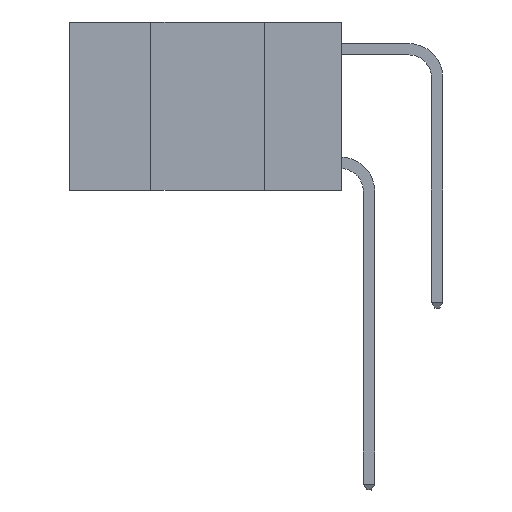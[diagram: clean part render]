
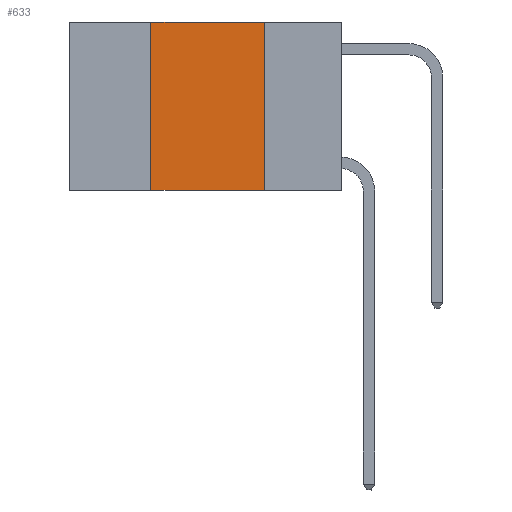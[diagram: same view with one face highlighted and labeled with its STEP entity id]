
A CAD part, left-side view. The second image highlights one B-rep face of the part: STEP entity #633.
In plain terms, the highlighted planar face has unit normal (-1, 0, 0).
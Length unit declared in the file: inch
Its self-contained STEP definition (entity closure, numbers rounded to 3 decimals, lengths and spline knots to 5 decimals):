
#192 = VECTOR ( 'NONE', #5449, 39.37008 ) ;
#633 = ADVANCED_FACE ( 'NONE', ( #22563 ), #10099, .F. ) ;
#636 = CARTESIAN_POINT ( 'NONE',  ( 0., 0.6, -0.37 ) ) ;
#1644 = DIRECTION ( 'NONE',  ( 0., 0., 1. ) ) ;
#1750 = LINE ( 'NONE', #636, #192 ) ;
#2427 = EDGE_CURVE ( 'NONE', #15193, #10401, #23964, .T. ) ;
#3331 = ORIENTED_EDGE ( 'NONE', *, *, #22176, .F. ) ;
#3996 = EDGE_CURVE ( 'NONE', #10401, #15810, #9473, .T. ) ;
#4990 = CARTESIAN_POINT ( 'NONE',  ( 0., 0.42, 0. ) ) ;
#5006 = CARTESIAN_POINT ( 'NONE',  ( 0., 0.6, 0. ) ) ;
#5449 = DIRECTION ( 'NONE',  ( 0., -1., 0. ) ) ;
#8804 = CARTESIAN_POINT ( 'NONE',  ( 0., 0.42, 0. ) ) ;
#9050 = CARTESIAN_POINT ( 'NONE',  ( 0., 0.42, -0.37 ) ) ;
#9473 = LINE ( 'NONE', #5006, #13579 ) ;
#9887 = DIRECTION ( 'NONE',  ( 1., 0., 0. ) ) ;
#10099 = PLANE ( 'NONE',  #14474 ) ;
#10401 = VERTEX_POINT ( 'NONE', #4990 ) ;
#10667 = EDGE_LOOP ( 'NONE', ( #3331, #27236, #23831, #16874 ) ) ;
#10698 = VECTOR ( 'NONE', #1644, 39.37008 ) ;
#10880 = VERTEX_POINT ( 'NONE', #19315 ) ;
#13579 = VECTOR ( 'NONE', #29328, 39.37008 ) ;
#13625 = CARTESIAN_POINT ( 'NONE',  ( 0., 0.17, 0. ) ) ;
#13937 = CARTESIAN_POINT ( 'NONE',  ( 0., 0.17, 0. ) ) ;
#14339 = DIRECTION ( 'NONE',  ( 0., 0., -1. ) ) ;
#14474 = AXIS2_PLACEMENT_3D ( 'NONE', #19930, #9887, #29342 ) ;
#15193 = VERTEX_POINT ( 'NONE', #9050 ) ;
#15810 = VERTEX_POINT ( 'NONE', #13625 ) ;
#16874 = ORIENTED_EDGE ( 'NONE', *, *, #19059, .T. ) ;
#18948 = LINE ( 'NONE', #13937, #28876 ) ;
#19059 = EDGE_CURVE ( 'NONE', #15193, #10880, #1750, .T. ) ;
#19315 = CARTESIAN_POINT ( 'NONE',  ( 0., 0.17, -0.37 ) ) ;
#19930 = CARTESIAN_POINT ( 'NONE',  ( 0., 0.6, 0. ) ) ;
#22176 = EDGE_CURVE ( 'NONE', #15810, #10880, #18948, .T. ) ;
#22563 = FACE_OUTER_BOUND ( 'NONE', #10667, .T. ) ;
#23831 = ORIENTED_EDGE ( 'NONE', *, *, #2427, .F. ) ;
#23964 = LINE ( 'NONE', #8804, #10698 ) ;
#27236 = ORIENTED_EDGE ( 'NONE', *, *, #3996, .F. ) ;
#28876 = VECTOR ( 'NONE', #14339, 39.37008 ) ;
#29328 = DIRECTION ( 'NONE',  ( 0., -1., 0. ) ) ;
#29342 = DIRECTION ( 'NONE',  ( 0., 0., -1. ) ) ;
